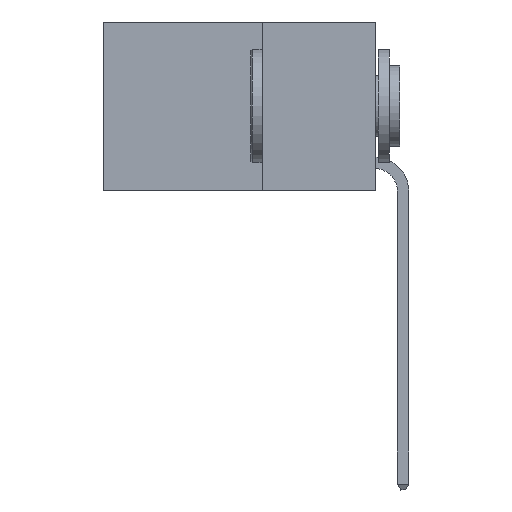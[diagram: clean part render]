
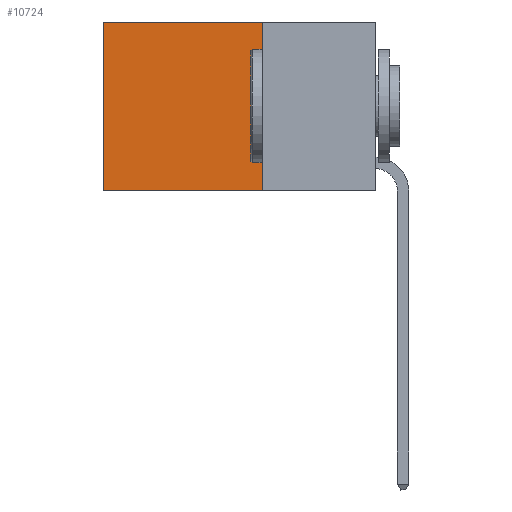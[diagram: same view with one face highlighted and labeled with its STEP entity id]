
A CAD part, left-side view. The second image highlights one B-rep face of the part: STEP entity #10724.
In plain terms, the highlighted planar face has unit normal (-1, 0, 0).
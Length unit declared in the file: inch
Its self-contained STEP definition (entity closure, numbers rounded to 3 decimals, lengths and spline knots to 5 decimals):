
#666 = EDGE_LOOP ( 'NONE', ( #25812, #8934, #10262, #14252 ) ) ;
#864 = VECTOR ( 'NONE', #3009, 39.37008 ) ;
#1799 = DIRECTION ( 'NONE',  ( 0., 0., -1. ) ) ;
#3009 = DIRECTION ( 'NONE',  ( 0., 0., -1. ) ) ;
#3210 = DIRECTION ( 'NONE',  ( 0., 0., -1. ) ) ;
#3772 = CARTESIAN_POINT ( 'NONE',  ( 0.2625, 0.25, 0. ) ) ;
#5186 = CARTESIAN_POINT ( 'NONE',  ( 0.2625, 0.25, 0. ) ) ;
#6140 = FACE_OUTER_BOUND ( 'NONE', #666, .T. ) ;
#6270 = DIRECTION ( 'NONE',  ( 1., 0., 0. ) ) ;
#7200 = LINE ( 'NONE', #5186, #864 ) ;
#7578 = CARTESIAN_POINT ( 'NONE',  ( 0.2625, 0.25, 0. ) ) ;
#8934 = ORIENTED_EDGE ( 'NONE', *, *, #20903, .F. ) ;
#9803 = EDGE_CURVE ( 'NONE', #21476, #26957, #23282, .T. ) ;
#10262 = ORIENTED_EDGE ( 'NONE', *, *, #15797, .F. ) ;
#10724 = ADVANCED_FACE ( 'NONE', ( #6140 ), #21720, .F. ) ;
#12712 = CARTESIAN_POINT ( 'NONE',  ( 0.2625, 0.25, 0. ) ) ;
#13317 = CARTESIAN_POINT ( 'NONE',  ( 0.2625, 0.25, -0.37 ) ) ;
#13754 = VERTEX_POINT ( 'NONE', #15300 ) ;
#14100 = EDGE_CURVE ( 'NONE', #19135, #21476, #25449, .T. ) ;
#14252 = ORIENTED_EDGE ( 'NONE', *, *, #14100, .T. ) ;
#15300 = CARTESIAN_POINT ( 'NONE',  ( 0.2625, 0.25, -0.37 ) ) ;
#15797 = EDGE_CURVE ( 'NONE', #19135, #13754, #7200, .T. ) ;
#19135 = VERTEX_POINT ( 'NONE', #7578 ) ;
#19366 = VECTOR ( 'NONE', #25593, 39.37008 ) ;
#20020 = DIRECTION ( 'NONE',  ( 0., 1., 0. ) ) ;
#20222 = VECTOR ( 'NONE', #3210, 39.37008 ) ;
#20796 = CARTESIAN_POINT ( 'NONE',  ( 0.2625, 0.6, 0. ) ) ;
#20903 = EDGE_CURVE ( 'NONE', #13754, #26957, #22343, .T. ) ;
#21476 = VERTEX_POINT ( 'NONE', #20796 ) ;
#21720 = PLANE ( 'NONE',  #27788 ) ;
#21904 = VECTOR ( 'NONE', #20020, 39.37008 ) ;
#22343 = LINE ( 'NONE', #13317, #21904 ) ;
#23282 = LINE ( 'NONE', #25601, #20222 ) ;
#25449 = LINE ( 'NONE', #3772, #19366 ) ;
#25593 = DIRECTION ( 'NONE',  ( 0., 1., 0. ) ) ;
#25601 = CARTESIAN_POINT ( 'NONE',  ( 0.2625, 0.6, 0. ) ) ;
#25812 = ORIENTED_EDGE ( 'NONE', *, *, #9803, .T. ) ;
#26957 = VERTEX_POINT ( 'NONE', #27148 ) ;
#27148 = CARTESIAN_POINT ( 'NONE',  ( 0.2625, 0.6, -0.37 ) ) ;
#27788 = AXIS2_PLACEMENT_3D ( 'NONE', #12712, #6270, #1799 ) ;
